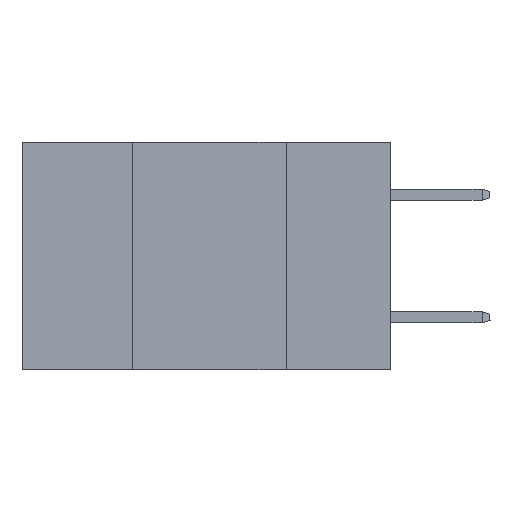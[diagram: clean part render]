
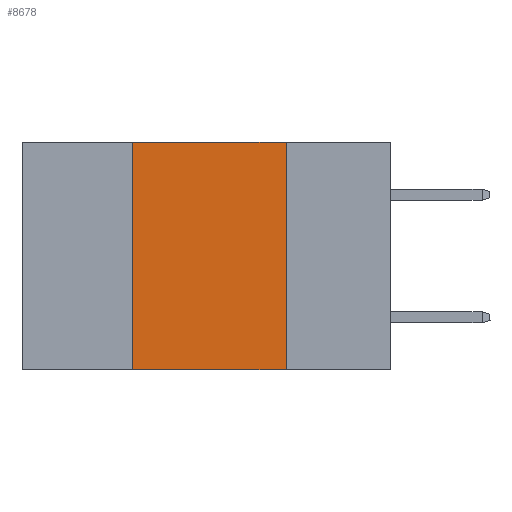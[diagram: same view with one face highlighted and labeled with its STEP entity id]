
A CAD part, left-side view. The second image highlights one B-rep face of the part: STEP entity #8678.
In plain terms, the highlighted planar face has unit normal (-1, 0, 0).
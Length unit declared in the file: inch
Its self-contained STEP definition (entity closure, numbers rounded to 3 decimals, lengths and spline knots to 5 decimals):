
#22 = VECTOR ( 'NONE', #18816, 39.37008 ) ;
#946 = CARTESIAN_POINT ( 'NONE',  ( 0., 0.6, 0. ) ) ;
#2530 = DIRECTION ( 'NONE',  ( 0., 0., 1. ) ) ;
#4074 = LINE ( 'NONE', #9645, #12349 ) ;
#4088 = CARTESIAN_POINT ( 'NONE',  ( 0., 0.6, 0. ) ) ;
#4204 = VECTOR ( 'NONE', #14208, 39.37008 ) ;
#4256 = LINE ( 'NONE', #6624, #22 ) ;
#4760 = LINE ( 'NONE', #8892, #4204 ) ;
#5164 = CARTESIAN_POINT ( 'NONE',  ( 0., 0.42, -0.37 ) ) ;
#5235 = EDGE_CURVE ( 'NONE', #5343, #18222, #4256, .T. ) ;
#5343 = VERTEX_POINT ( 'NONE', #5164 ) ;
#6226 = DIRECTION ( 'NONE',  ( 0., -1., 0. ) ) ;
#6624 = CARTESIAN_POINT ( 'NONE',  ( 0., 0.6, -0.37 ) ) ;
#7653 = DIRECTION ( 'NONE',  ( 1., 0., 0. ) ) ;
#7964 = VECTOR ( 'NONE', #6226, 39.37008 ) ;
#8070 = CARTESIAN_POINT ( 'NONE',  ( 0., 0.17, -0.37 ) ) ;
#8678 = ADVANCED_FACE ( 'NONE', ( #10143 ), #18041, .F. ) ;
#8876 = EDGE_CURVE ( 'NONE', #10660, #15394, #21256, .T. ) ;
#8892 = CARTESIAN_POINT ( 'NONE',  ( 0., 0.17, 0. ) ) ;
#9645 = CARTESIAN_POINT ( 'NONE',  ( 0., 0.42, 0. ) ) ;
#10143 = FACE_OUTER_BOUND ( 'NONE', #18975, .T. ) ;
#10373 = AXIS2_PLACEMENT_3D ( 'NONE', #4088, #7653, #19820 ) ;
#10660 = VERTEX_POINT ( 'NONE', #14786 ) ;
#12349 = VECTOR ( 'NONE', #2530, 39.37008 ) ;
#14208 = DIRECTION ( 'NONE',  ( 0., 0., -1. ) ) ;
#14470 = CARTESIAN_POINT ( 'NONE',  ( 0., 0.17, 0. ) ) ;
#14786 = CARTESIAN_POINT ( 'NONE',  ( 0., 0.42, 0. ) ) ;
#15394 = VERTEX_POINT ( 'NONE', #14470 ) ;
#18041 = PLANE ( 'NONE',  #10373 ) ;
#18222 = VERTEX_POINT ( 'NONE', #8070 ) ;
#18473 = ORIENTED_EDGE ( 'NONE', *, *, #18515, .F. ) ;
#18515 = EDGE_CURVE ( 'NONE', #15394, #18222, #4760, .T. ) ;
#18516 = ORIENTED_EDGE ( 'NONE', *, *, #8876, .F. ) ;
#18677 = ORIENTED_EDGE ( 'NONE', *, *, #21959, .F. ) ;
#18699 = ORIENTED_EDGE ( 'NONE', *, *, #5235, .T. ) ;
#18816 = DIRECTION ( 'NONE',  ( 0., -1., 0. ) ) ;
#18975 = EDGE_LOOP ( 'NONE', ( #18473, #18516, #18677, #18699 ) ) ;
#19820 = DIRECTION ( 'NONE',  ( 0., 0., -1. ) ) ;
#21256 = LINE ( 'NONE', #946, #7964 ) ;
#21959 = EDGE_CURVE ( 'NONE', #5343, #10660, #4074, .T. ) ;
